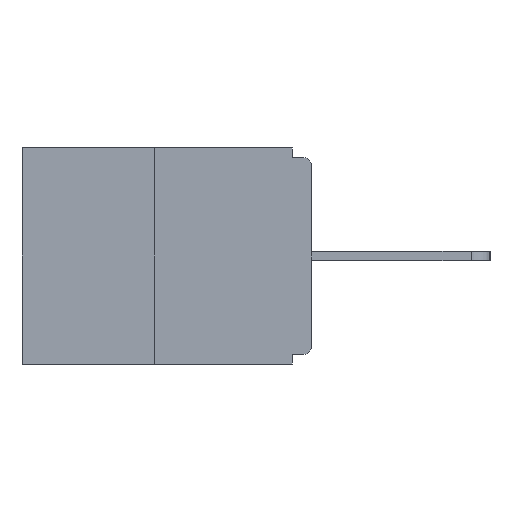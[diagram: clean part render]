
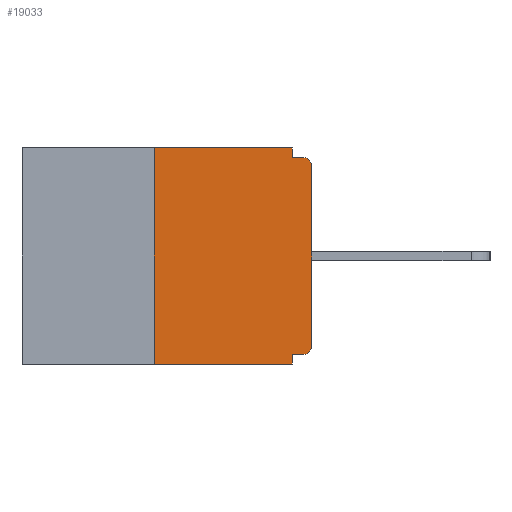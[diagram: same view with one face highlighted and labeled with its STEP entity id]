
A CAD part, left-side view. The second image highlights one B-rep face of the part: STEP entity #19033.
In plain terms, the highlighted planar face has unit normal (-1, 0, 0).
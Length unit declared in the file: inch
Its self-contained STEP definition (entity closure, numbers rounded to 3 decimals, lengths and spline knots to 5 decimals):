
#508 = DIRECTION ( 'NONE',  ( 0., -1., 0. ) ) ;
#1753 = LINE ( 'NONE', #22047, #19451 ) ;
#2152 = VERTEX_POINT ( 'NONE', #14079 ) ;
#2245 = VECTOR ( 'NONE', #23393, 39.37008 ) ;
#2394 = VERTEX_POINT ( 'NONE', #24073 ) ;
#2415 = VECTOR ( 'NONE', #2527, 39.37008 ) ;
#2527 = DIRECTION ( 'NONE',  ( 0., 1., 0. ) ) ;
#2603 = EDGE_CURVE ( 'NONE', #2152, #9390, #23309, .T. ) ;
#2724 = EDGE_CURVE ( 'NONE', #11450, #19790, #1753, .T. ) ;
#2773 = VECTOR ( 'NONE', #16992, 39.37008 ) ;
#2853 = LINE ( 'NONE', #14394, #6017 ) ;
#3830 = CARTESIAN_POINT ( 'NONE',  ( 0., 0.46, 0. ) ) ;
#4222 = DIRECTION ( 'NONE',  ( -1., 0., 0. ) ) ;
#4332 = CIRCLE ( 'NONE', #19798, 0.015 ) ;
#4433 = DIRECTION ( 'NONE',  ( 0., -1., 0. ) ) ;
#4468 = CARTESIAN_POINT ( 'NONE',  ( 0., 0., -0.328 ) ) ;
#4498 = EDGE_CURVE ( 'NONE', #19790, #8231, #2853, .T. ) ;
#4524 = CARTESIAN_POINT ( 'NONE',  ( 0., 0.031, -0.343 ) ) ;
#4896 = VECTOR ( 'NONE', #508, 39.37008 ) ;
#5064 = ORIENTED_EDGE ( 'NONE', *, *, #15200, .T. ) ;
#5781 = CIRCLE ( 'NONE', #20038, 0.015 ) ;
#5826 = DIRECTION ( 'NONE',  ( 0., 0., -1. ) ) ;
#5939 = LINE ( 'NONE', #22921, #2773 ) ;
#6017 = VECTOR ( 'NONE', #4433, 39.37008 ) ;
#6888 = ORIENTED_EDGE ( 'NONE', *, *, #13951, .F. ) ;
#7187 = CARTESIAN_POINT ( 'NONE',  ( 0., 0., -0.313 ) ) ;
#7496 = CARTESIAN_POINT ( 'NONE',  ( 0., 0.015, -0.328 ) ) ;
#8231 = VERTEX_POINT ( 'NONE', #22259 ) ;
#8311 = ORIENTED_EDGE ( 'NONE', *, *, #2724, .F. ) ;
#8351 = LINE ( 'NONE', #4468, #2415 ) ;
#9086 = CARTESIAN_POINT ( 'NONE',  ( 0., 0.031, -0.343 ) ) ;
#9315 = FACE_OUTER_BOUND ( 'NONE', #13581, .T. ) ;
#9390 = VERTEX_POINT ( 'NONE', #14570 ) ;
#9937 = LINE ( 'NONE', #17256, #4896 ) ;
#10013 = EDGE_CURVE ( 'NONE', #11755, #8231, #4332, .T. ) ;
#10437 = CARTESIAN_POINT ( 'NONE',  ( 0., 0.25, 0. ) ) ;
#11169 = ORIENTED_EDGE ( 'NONE', *, *, #10013, .T. ) ;
#11450 = VERTEX_POINT ( 'NONE', #14650 ) ;
#11577 = ORIENTED_EDGE ( 'NONE', *, *, #15523, .F. ) ;
#11755 = VERTEX_POINT ( 'NONE', #14247 ) ;
#12217 = ORIENTED_EDGE ( 'NONE', *, *, #22771, .F. ) ;
#13032 = DIRECTION ( 'NONE',  ( 0., 0., -1. ) ) ;
#13415 = AXIS2_PLACEMENT_3D ( 'NONE', #3830, #23048, #13032 ) ;
#13581 = EDGE_LOOP ( 'NONE', ( #6888, #17752, #22059, #11577, #12217, #5064, #20600, #11169, #21929, #8311 ) ) ;
#13678 = CARTESIAN_POINT ( 'NONE',  ( 0., 0.015, -0.313 ) ) ;
#13834 = EDGE_CURVE ( 'NONE', #22105, #11755, #18488, .T. ) ;
#13951 = EDGE_CURVE ( 'NONE', #9390, #11450, #9937, .T. ) ;
#14079 = CARTESIAN_POINT ( 'NONE',  ( 0., 0.25, -0.343 ) ) ;
#14247 = CARTESIAN_POINT ( 'NONE',  ( 0., 0., -0.03 ) ) ;
#14394 = CARTESIAN_POINT ( 'NONE',  ( 0., 0., -0.015 ) ) ;
#14414 = DIRECTION ( 'NONE',  ( 0., 0., 1. ) ) ;
#14570 = CARTESIAN_POINT ( 'NONE',  ( 0., 0.25, 0. ) ) ;
#14650 = CARTESIAN_POINT ( 'NONE',  ( 0., 0.031, 0. ) ) ;
#15200 = EDGE_CURVE ( 'NONE', #16250, #22105, #5781, .T. ) ;
#15523 = EDGE_CURVE ( 'NONE', #2394, #16807, #17599, .T. ) ;
#16250 = VERTEX_POINT ( 'NONE', #7496 ) ;
#16388 = DIRECTION ( 'NONE',  ( 0., 0., -1. ) ) ;
#16696 = VECTOR ( 'NONE', #14414, 39.37008 ) ;
#16807 = VERTEX_POINT ( 'NONE', #9086 ) ;
#16870 = PLANE ( 'NONE',  #13415 ) ;
#16992 = DIRECTION ( 'NONE',  ( 0., -1., 0. ) ) ;
#17256 = CARTESIAN_POINT ( 'NONE',  ( 0., 0.46, 0. ) ) ;
#17517 = CARTESIAN_POINT ( 'NONE',  ( 0., 0.015, -0.03 ) ) ;
#17599 = LINE ( 'NONE', #4524, #2245 ) ;
#17653 = DIRECTION ( 'NONE',  ( 0., 0., -1. ) ) ;
#17752 = ORIENTED_EDGE ( 'NONE', *, *, #2603, .F. ) ;
#18488 = LINE ( 'NONE', #22317, #19179 ) ;
#18943 = EDGE_CURVE ( 'NONE', #2152, #16807, #5939, .T. ) ;
#19033 = ADVANCED_FACE ( 'NONE', ( #9315 ), #16870, .F. ) ;
#19049 = CARTESIAN_POINT ( 'NONE',  ( 0., 0.031, -0.015 ) ) ;
#19179 = VECTOR ( 'NONE', #24427, 39.37008 ) ;
#19451 = VECTOR ( 'NONE', #16388, 39.37008 ) ;
#19790 = VERTEX_POINT ( 'NONE', #19049 ) ;
#19798 = AXIS2_PLACEMENT_3D ( 'NONE', #17517, #22815, #5826 ) ;
#20038 = AXIS2_PLACEMENT_3D ( 'NONE', #13678, #4222, #17653 ) ;
#20600 = ORIENTED_EDGE ( 'NONE', *, *, #13834, .T. ) ;
#21929 = ORIENTED_EDGE ( 'NONE', *, *, #4498, .F. ) ;
#22047 = CARTESIAN_POINT ( 'NONE',  ( 0., 0.031, 0. ) ) ;
#22059 = ORIENTED_EDGE ( 'NONE', *, *, #18943, .T. ) ;
#22105 = VERTEX_POINT ( 'NONE', #7187 ) ;
#22259 = CARTESIAN_POINT ( 'NONE',  ( 0., 0.015, -0.015 ) ) ;
#22317 = CARTESIAN_POINT ( 'NONE',  ( 0., 0., 0. ) ) ;
#22771 = EDGE_CURVE ( 'NONE', #16250, #2394, #8351, .T. ) ;
#22815 = DIRECTION ( 'NONE',  ( -1., 0., 0. ) ) ;
#22921 = CARTESIAN_POINT ( 'NONE',  ( 0., 0.46, -0.343 ) ) ;
#23048 = DIRECTION ( 'NONE',  ( 1., 0., 0. ) ) ;
#23309 = LINE ( 'NONE', #10437, #16696 ) ;
#23393 = DIRECTION ( 'NONE',  ( 0., 0., -1. ) ) ;
#24073 = CARTESIAN_POINT ( 'NONE',  ( 0., 0.031, -0.328 ) ) ;
#24427 = DIRECTION ( 'NONE',  ( 0., 0., 1. ) ) ;
